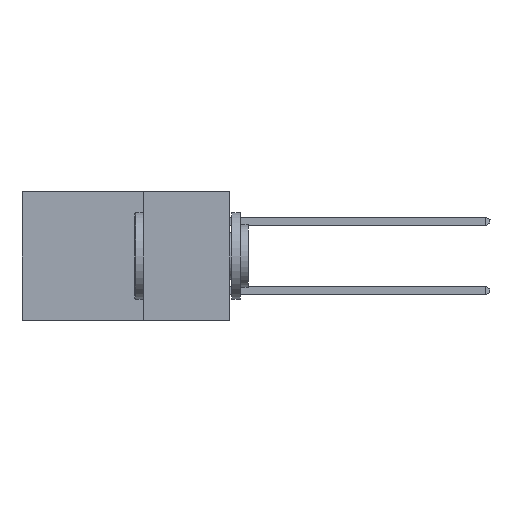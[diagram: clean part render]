
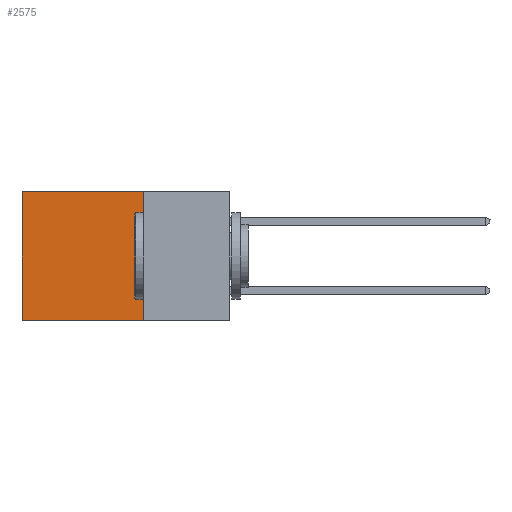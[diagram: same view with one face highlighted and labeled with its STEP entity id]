
A CAD part, left-side view. The second image highlights one B-rep face of the part: STEP entity #2575.
In plain terms, the highlighted planar face has unit normal (-1, 0, 0).
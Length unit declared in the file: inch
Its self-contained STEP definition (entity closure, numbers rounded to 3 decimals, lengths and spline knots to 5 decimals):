
#27 = CARTESIAN_POINT ( 'NONE',  ( 0.2615, 0.25, -0.37 ) ) ;
#464 = DIRECTION ( 'NONE',  ( 0., 0., -1. ) ) ;
#484 = VECTOR ( 'NONE', #4584, 39.37008 ) ;
#726 = VECTOR ( 'NONE', #10354, 39.37008 ) ;
#833 = CARTESIAN_POINT ( 'NONE',  ( 0.2615, 0.6, -0.37 ) ) ;
#1966 = ORIENTED_EDGE ( 'NONE', *, *, #2524, .F. ) ;
#2330 = LINE ( 'NONE', #27, #726 ) ;
#2496 = CARTESIAN_POINT ( 'NONE',  ( 0.2615, 0.25, -0.37 ) ) ;
#2524 = EDGE_CURVE ( 'NONE', #5370, #7276, #8615, .T. ) ;
#2572 = PLANE ( 'NONE',  #8564 ) ;
#2575 = ADVANCED_FACE ( 'NONE', ( #10723 ), #2572, .F. ) ;
#2645 = CARTESIAN_POINT ( 'NONE',  ( 0.2615, 0.25, 0. ) ) ;
#3469 = ORIENTED_EDGE ( 'NONE', *, *, #6161, .T. ) ;
#3588 = LINE ( 'NONE', #2645, #484 ) ;
#4025 = CARTESIAN_POINT ( 'NONE',  ( 0.2615, 0.6, 0. ) ) ;
#4326 = VERTEX_POINT ( 'NONE', #8601 ) ;
#4448 = DIRECTION ( 'NONE',  ( 1., 0., 0. ) ) ;
#4578 = DIRECTION ( 'NONE',  ( 0., 1., 0. ) ) ;
#4584 = DIRECTION ( 'NONE',  ( 0., 1., 0. ) ) ;
#5328 = VECTOR ( 'NONE', #4578, 39.37008 ) ;
#5370 = VERTEX_POINT ( 'NONE', #10085 ) ;
#5390 = CARTESIAN_POINT ( 'NONE',  ( 0.2615, 0.25, -0.37 ) ) ;
#6161 = EDGE_CURVE ( 'NONE', #4326, #8554, #3588, .T. ) ;
#7181 = EDGE_LOOP ( 'NONE', ( #8929, #1966, #10122, #3469 ) ) ;
#7276 = VERTEX_POINT ( 'NONE', #833 ) ;
#7365 = CARTESIAN_POINT ( 'NONE',  ( 0.2615, 0.6, -0.37 ) ) ;
#8130 = EDGE_CURVE ( 'NONE', #4326, #5370, #2330, .T. ) ;
#8436 = DIRECTION ( 'NONE',  ( 0., 0., -1. ) ) ;
#8554 = VERTEX_POINT ( 'NONE', #4025 ) ;
#8564 = AXIS2_PLACEMENT_3D ( 'NONE', #2496, #4448, #464 ) ;
#8601 = CARTESIAN_POINT ( 'NONE',  ( 0.2615, 0.25, 0. ) ) ;
#8615 = LINE ( 'NONE', #5390, #5328 ) ;
#8646 = EDGE_CURVE ( 'NONE', #8554, #7276, #10335, .T. ) ;
#8929 = ORIENTED_EDGE ( 'NONE', *, *, #8646, .T. ) ;
#9780 = VECTOR ( 'NONE', #8436, 39.37008 ) ;
#10085 = CARTESIAN_POINT ( 'NONE',  ( 0.2615, 0.25, -0.37 ) ) ;
#10122 = ORIENTED_EDGE ( 'NONE', *, *, #8130, .F. ) ;
#10335 = LINE ( 'NONE', #7365, #9780 ) ;
#10354 = DIRECTION ( 'NONE',  ( 0., 0., -1. ) ) ;
#10723 = FACE_OUTER_BOUND ( 'NONE', #7181, .T. ) ;
